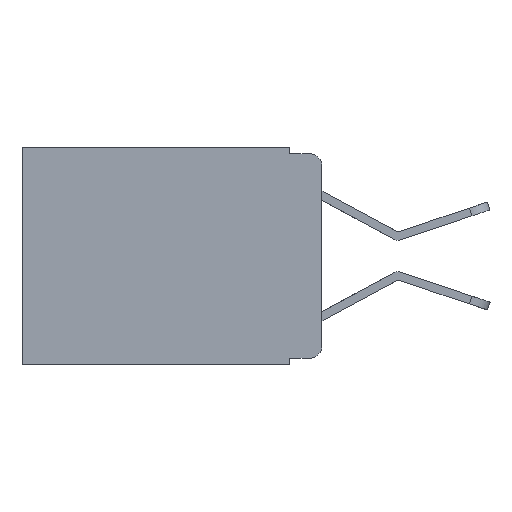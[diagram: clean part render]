
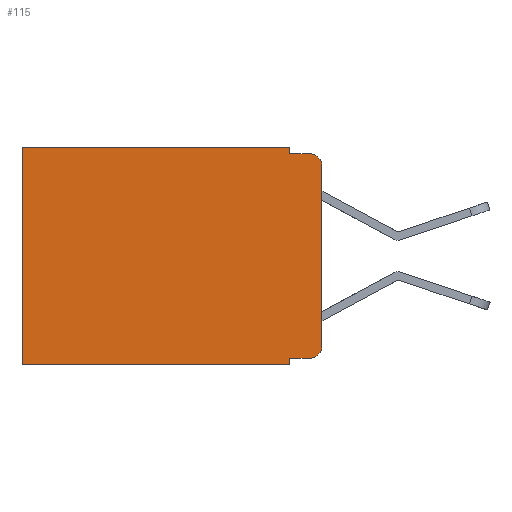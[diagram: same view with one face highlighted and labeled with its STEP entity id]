
A CAD part, left-side view. The second image highlights one B-rep face of the part: STEP entity #115.
In plain terms, the highlighted planar face has unit normal (-1, 0, 0).
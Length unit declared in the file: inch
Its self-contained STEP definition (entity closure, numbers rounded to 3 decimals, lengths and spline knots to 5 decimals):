
#115 = ADVANCED_FACE ( 'NONE', ( #2238 ), #5369, .F. ) ;
#131 = VECTOR ( 'NONE', #491, 39.37008 ) ;
#167 = ORIENTED_EDGE ( 'NONE', *, *, #4021, .T. ) ;
#200 = EDGE_CURVE ( 'NONE', #9953, #12453, #13637, .T. ) ;
#394 = LINE ( 'NONE', #12239, #8819 ) ;
#491 = DIRECTION ( 'NONE',  ( 0., 1., 0. ) ) ;
#1057 = CARTESIAN_POINT ( 'NONE',  ( 0.298, 0.051, 0. ) ) ;
#1359 = DIRECTION ( 'NONE',  ( -1., 0., 0. ) ) ;
#1809 = EDGE_CURVE ( 'NONE', #6697, #3428, #4597, .T. ) ;
#1828 = CARTESIAN_POINT ( 'NONE',  ( 0.298, 0.02, -0.333 ) ) ;
#1868 = DIRECTION ( 'NONE',  ( 0., 0., -1. ) ) ;
#1945 = VECTOR ( 'NONE', #9336, 39.37008 ) ;
#2126 = ORIENTED_EDGE ( 'NONE', *, *, #1809, .T. ) ;
#2142 = DIRECTION ( 'NONE',  ( -1., 0., 0. ) ) ;
#2238 = FACE_OUTER_BOUND ( 'NONE', #10961, .T. ) ;
#2502 = EDGE_CURVE ( 'NONE', #10195, #10050, #3168, .T. ) ;
#2562 = EDGE_CURVE ( 'NONE', #13261, #10050, #13811, .T. ) ;
#2596 = LINE ( 'NONE', #2792, #131 ) ;
#2792 = CARTESIAN_POINT ( 'NONE',  ( 0.298, 0., -0.343 ) ) ;
#3164 = VERTEX_POINT ( 'NONE', #5805 ) ;
#3168 = LINE ( 'NONE', #4144, #5719 ) ;
#3195 = EDGE_CURVE ( 'NONE', #12124, #3428, #2596, .T. ) ;
#3275 = DIRECTION ( 'NONE',  ( 0., 0., -1. ) ) ;
#3280 = VERTEX_POINT ( 'NONE', #10651 ) ;
#3319 = LINE ( 'NONE', #7610, #9159 ) ;
#3348 = VECTOR ( 'NONE', #1868, 39.37008 ) ;
#3428 = VERTEX_POINT ( 'NONE', #4519 ) ;
#3459 = EDGE_CURVE ( 'NONE', #13261, #12453, #6498, .T. ) ;
#4021 = EDGE_CURVE ( 'NONE', #3280, #6697, #10203, .T. ) ;
#4144 = CARTESIAN_POINT ( 'NONE',  ( 0.298, 0.051, -0.01 ) ) ;
#4319 = CARTESIAN_POINT ( 'NONE',  ( 0.298, 0., 0. ) ) ;
#4519 = CARTESIAN_POINT ( 'NONE',  ( 0.298, 0.473, -0.343 ) ) ;
#4543 = ORIENTED_EDGE ( 'NONE', *, *, #5789, .T. ) ;
#4597 = LINE ( 'NONE', #10367, #3348 ) ;
#4612 = AXIS2_PLACEMENT_3D ( 'NONE', #4319, #8618, #3275 ) ;
#4733 = EDGE_CURVE ( 'NONE', #3280, #10195, #8416, .T. ) ;
#4763 = CARTESIAN_POINT ( 'NONE',  ( 0.298, 0., 0. ) ) ;
#5094 = ORIENTED_EDGE ( 'NONE', *, *, #4733, .F. ) ;
#5166 = DIRECTION ( 'NONE',  ( 0., 0., -1. ) ) ;
#5306 = VECTOR ( 'NONE', #5166, 39.37008 ) ;
#5369 = PLANE ( 'NONE',  #4612 ) ;
#5406 = CARTESIAN_POINT ( 'NONE',  ( 0.298, 0.02, -0.03 ) ) ;
#5719 = VECTOR ( 'NONE', #8438, 39.37008 ) ;
#5789 = EDGE_CURVE ( 'NONE', #3164, #9953, #3319, .T. ) ;
#5805 = CARTESIAN_POINT ( 'NONE',  ( 0.298, 0.051, -0.333 ) ) ;
#6003 = CARTESIAN_POINT ( 'NONE',  ( 0.298, 0.051, -0.01 ) ) ;
#6122 = CARTESIAN_POINT ( 'NONE',  ( 0.298, 0.02, -0.313 ) ) ;
#6498 = LINE ( 'NONE', #6634, #10018 ) ;
#6634 = CARTESIAN_POINT ( 'NONE',  ( 0.298, 0., 0. ) ) ;
#6697 = VERTEX_POINT ( 'NONE', #7493 ) ;
#6836 = ORIENTED_EDGE ( 'NONE', *, *, #3195, .F. ) ;
#7056 = AXIS2_PLACEMENT_3D ( 'NONE', #5406, #1359, #8719 ) ;
#7493 = CARTESIAN_POINT ( 'NONE',  ( 0.298, 0.473, 0. ) ) ;
#7571 = ORIENTED_EDGE ( 'NONE', *, *, #3459, .F. ) ;
#7610 = CARTESIAN_POINT ( 'NONE',  ( 0.298, 0.051, -0.333 ) ) ;
#8013 = CARTESIAN_POINT ( 'NONE',  ( 0.298, 0., -0.03 ) ) ;
#8416 = LINE ( 'NONE', #1057, #5306 ) ;
#8438 = DIRECTION ( 'NONE',  ( 0., -1., 0. ) ) ;
#8601 = CARTESIAN_POINT ( 'NONE',  ( 0.298, 0.051, -0.343 ) ) ;
#8618 = DIRECTION ( 'NONE',  ( 1., 0., 0. ) ) ;
#8719 = DIRECTION ( 'NONE',  ( 0., 0., -1. ) ) ;
#8819 = VECTOR ( 'NONE', #8953, 39.37008 ) ;
#8953 = DIRECTION ( 'NONE',  ( 0., 0., -1. ) ) ;
#9073 = ORIENTED_EDGE ( 'NONE', *, *, #200, .T. ) ;
#9159 = VECTOR ( 'NONE', #12809, 39.37008 ) ;
#9292 = DIRECTION ( 'NONE',  ( 0., 0., -1. ) ) ;
#9336 = DIRECTION ( 'NONE',  ( 0., 1., 0. ) ) ;
#9685 = CARTESIAN_POINT ( 'NONE',  ( 0.298, 0.02, -0.01 ) ) ;
#9887 = DIRECTION ( 'NONE',  ( 0., 0., -1. ) ) ;
#9953 = VERTEX_POINT ( 'NONE', #1828 ) ;
#10018 = VECTOR ( 'NONE', #9887, 39.37008 ) ;
#10022 = ORIENTED_EDGE ( 'NONE', *, *, #2562, .T. ) ;
#10050 = VERTEX_POINT ( 'NONE', #9685 ) ;
#10096 = ORIENTED_EDGE ( 'NONE', *, *, #2502, .F. ) ;
#10195 = VERTEX_POINT ( 'NONE', #6003 ) ;
#10203 = LINE ( 'NONE', #4763, #1945 ) ;
#10367 = CARTESIAN_POINT ( 'NONE',  ( 0.298, 0.473, 0. ) ) ;
#10651 = CARTESIAN_POINT ( 'NONE',  ( 0.298, 0.051, 0. ) ) ;
#10961 = EDGE_LOOP ( 'NONE', ( #7571, #10022, #10096, #5094, #167, #2126, #6836, #12711, #4543, #9073 ) ) ;
#11668 = CARTESIAN_POINT ( 'NONE',  ( 0.298, 0., -0.313 ) ) ;
#12124 = VERTEX_POINT ( 'NONE', #8601 ) ;
#12230 = EDGE_CURVE ( 'NONE', #3164, #12124, #394, .T. ) ;
#12239 = CARTESIAN_POINT ( 'NONE',  ( 0.298, 0.051, 0. ) ) ;
#12453 = VERTEX_POINT ( 'NONE', #11668 ) ;
#12711 = ORIENTED_EDGE ( 'NONE', *, *, #12230, .F. ) ;
#12809 = DIRECTION ( 'NONE',  ( 0., -1., 0. ) ) ;
#12958 = AXIS2_PLACEMENT_3D ( 'NONE', #6122, #2142, #9292 ) ;
#13261 = VERTEX_POINT ( 'NONE', #8013 ) ;
#13637 = CIRCLE ( 'NONE', #12958, 0.02 ) ;
#13811 = CIRCLE ( 'NONE', #7056, 0.02 ) ;
